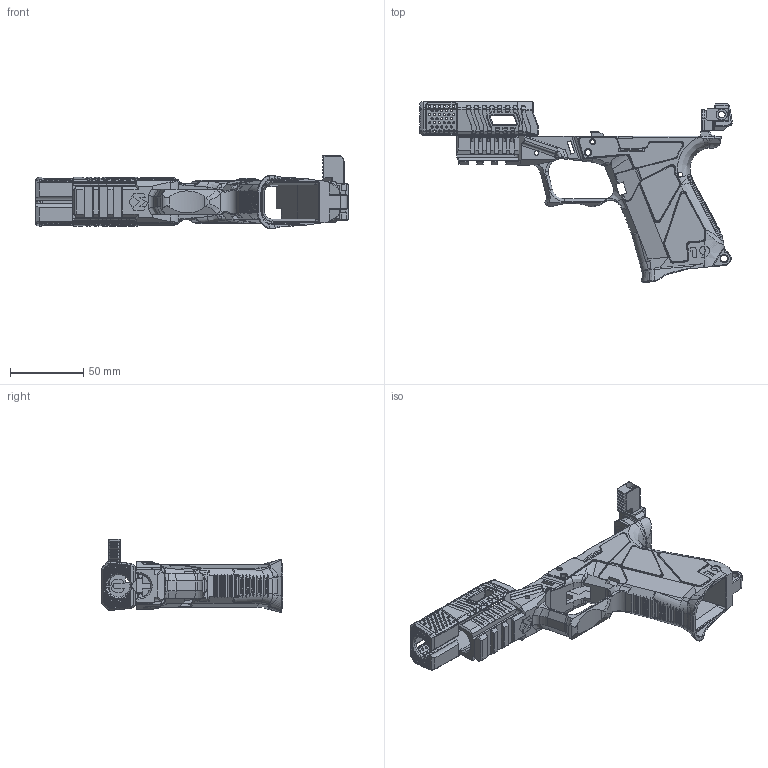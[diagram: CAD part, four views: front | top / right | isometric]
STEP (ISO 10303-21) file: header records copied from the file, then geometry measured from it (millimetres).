
FILE_DESCRIPTION (( 'STEP AP214' ), '1' );
FILE_NAME ('Schnitzel v1-5 Kit STEP.STEP', '2022-10-12T03:30:55', ( '' ), ( '' ), 'SwSTEP 2.0', 'SolidWorks 2020', '' );
FILE_SCHEMA (( 'AUTOMOTIVE_DESIGN' ));
Length unit declared in the file: inch
Products named in the file (4): Schnitzel v1-5 Kit STEP; Clamp Comp^KitAssem; Glock Charging Handle; r2
Assembly tree (3 placements, depth 2):
  Schnitzel v1-5 Kit STEP
    r2
    Clamp Comp^KitAssem
    Glock Charging Handle
Bounding box: 213.74 x 124.06 x 50.13 mm (x, y, z)
Volume: 111929 mm3; surface area: 66933.3 mm2
Topology: 4 solids, 7 shells, 3016 faces, 8383 edges, 5336 vertices
Faces by surface type: plane 1227, cylinder 857, bspline 689, cone 137, torus 86, sphere 20
Entity records: 133065 total; most frequent: CARTESIAN_POINT 62954, ORIENTED_EDGE 16756, DIRECTION 11466, EDGE_CURVE 8378, VERTEX_POINT 5336, LINE 4038, VECTOR 4038, AXIS2_PLACEMENT_3D 3714
